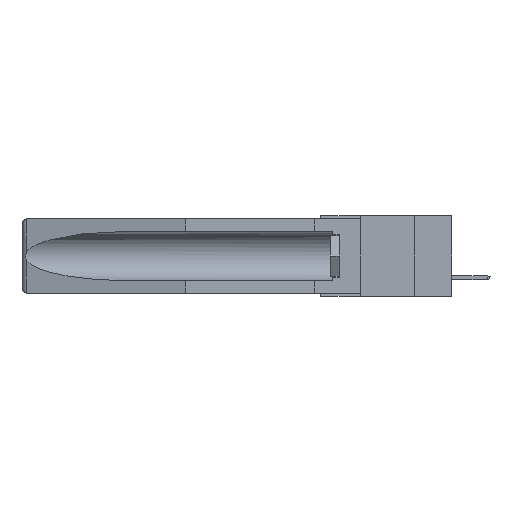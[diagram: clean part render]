
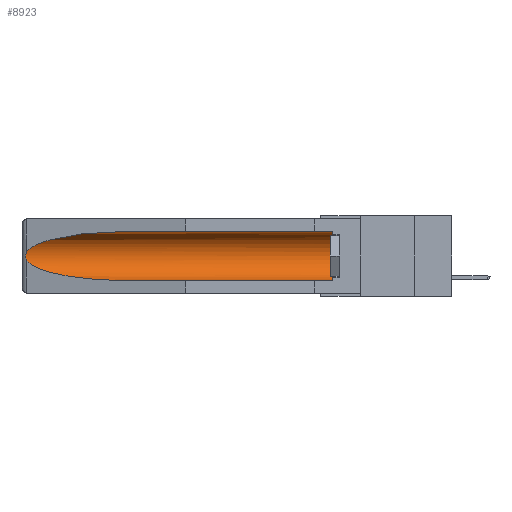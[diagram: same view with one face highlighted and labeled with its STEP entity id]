
A CAD part, left-side view. The second image highlights one B-rep face of the part: STEP entity #8923.
In plain terms, the highlighted cylindrical face has radius 2.857 mm (diameter 5.715 mm), a partial arc.
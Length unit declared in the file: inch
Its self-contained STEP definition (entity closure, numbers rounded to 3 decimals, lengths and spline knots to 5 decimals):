
#1051 = CARTESIAN_POINT ( 'NONE',  ( 0.2673, 1.5327, -0.16383 ) ) ;
#2566 = LINE ( 'NONE', #21143, #23350 ) ;
#3014 = VERTEX_POINT ( 'NONE', #20206 ) ;
#3257 = CARTESIAN_POINT ( 'NONE',  ( 0.26537, 1.52718, -0.19328 ) ) ;
#3435 = CARTESIAN_POINT ( 'NONE',  ( 0.26537, 1.52718, -0.14972 ) ) ;
#4205 = CARTESIAN_POINT ( 'NONE',  ( 0.26537, 1.52718, -0.14972 ) ) ;
#4552 = ORIENTED_EDGE ( 'NONE', *, *, #18517, .T. ) ;
#4690 = VERTEX_POINT ( 'NONE', #9397 ) ;
#5372 = CARTESIAN_POINT ( 'NONE',  ( 0.155, 0.126, -0.059 ) ) ;
#5679 = CARTESIAN_POINT ( 'NONE',  ( 0.26597, 1.5296, -0.19026 ) ) ;
#5900 = DIRECTION ( 'NONE',  ( 0., 1., 0. ) ) ;
#6109 = AXIS2_PLACEMENT_3D ( 'NONE', #16629, #5900, #23054 ) ;
#6149 = AXIS2_PLACEMENT_3D ( 'NONE', #6812, #26758, #14187 ) ;
#6570 = CARTESIAN_POINT ( 'NONE',  ( 0.155, 1.07973, -0.284 ) ) ;
#6812 = CARTESIAN_POINT ( 'NONE',  ( 0.155, 0.126, -0.1715 ) ) ;
#7363 = CARTESIAN_POINT ( 'NONE',  ( 0.26597, 1.52961, -0.15275 ) ) ;
#7870 = VERTEX_POINT ( 'NONE', #6570 ) ;
#7963 = VERTEX_POINT ( 'NONE', #15743 ) ;
#8196 =( BOUNDED_CURVE ( )  B_SPLINE_CURVE ( 3, ( #14705, #23470, #21165, #4205 ),
 .UNSPECIFIED., .F., .F. ) 
 B_SPLINE_CURVE_WITH_KNOTS ( ( 4, 4 ),
 ( 4.71239, 6.08839 ),
 .UNSPECIFIED. ) 
 CURVE ( )  GEOMETRIC_REPRESENTATION_ITEM ( )  RATIONAL_B_SPLINE_CURVE ( ( 1., 0.848, 0.848, 1. ) ) 
 REPRESENTATION_ITEM ( '' )  );
#8923 = ADVANCED_FACE ( 'NONE', ( #19555 ), #13847, .F. ) ;
#9397 = CARTESIAN_POINT ( 'NONE',  ( 0.155, 0.126, -0.284 ) ) ;
#9879 = CARTESIAN_POINT ( 'NONE',  ( 0.2675, 1.53308, -0.16763 ) ) ;
#10232 = EDGE_LOOP ( 'NONE', ( #20645, #14268, #4552, #20468, #12966, #24654 ) ) ;
#11658 = EDGE_CURVE ( 'NONE', #4690, #19636, #20367, .T. ) ;
#12394 = CARTESIAN_POINT ( 'NONE',  ( 0.25451, 1.48313, -0.24835 ) ) ;
#12966 = ORIENTED_EDGE ( 'NONE', *, *, #11658, .T. ) ;
#13592 = VECTOR ( 'NONE', #20528, 39.37008 ) ;
#13847 = CYLINDRICAL_SURFACE ( 'NONE', #6109, 0.1125 ) ;
#14187 = DIRECTION ( 'NONE',  ( 0., 0., 1. ) ) ;
#14268 = ORIENTED_EDGE ( 'NONE', *, *, #18723, .T. ) ;
#14344 = CARTESIAN_POINT ( 'NONE',  ( 0.155, -0.30754, -0.059 ) ) ;
#14534 = CARTESIAN_POINT ( 'NONE',  ( 0.155, 1.07973, -0.284 ) ) ;
#14582 = EDGE_CURVE ( 'NONE', #3014, #7963, #8196, .T. ) ;
#14705 = CARTESIAN_POINT ( 'NONE',  ( 0.155, 1.07973, -0.059 ) ) ;
#15743 = CARTESIAN_POINT ( 'NONE',  ( 0.26537, 1.52718, -0.14972 ) ) ;
#15986 = EDGE_CURVE ( 'NONE', #19636, #3014, #27618, .T. ) ;
#16610 = VERTEX_POINT ( 'NONE', #25281 ) ;
#16629 = CARTESIAN_POINT ( 'NONE',  ( 0.155, -0.30754, -0.1715 ) ) ;
#16876 = DIRECTION ( 'NONE',  ( 0., 1., 0. ) ) ;
#18517 = EDGE_CURVE ( 'NONE', #16610, #7870, #27719, .T. ) ;
#18723 = EDGE_CURVE ( 'NONE', #7963, #16610, #22783, .T. ) ;
#19555 = FACE_OUTER_BOUND ( 'NONE', #10232, .T. ) ;
#19636 = VERTEX_POINT ( 'NONE', #5372 ) ;
#20206 = CARTESIAN_POINT ( 'NONE',  ( 0.155, 1.07973, -0.059 ) ) ;
#20367 = CIRCLE ( 'NONE', #6149, 0.1125 ) ;
#20468 = ORIENTED_EDGE ( 'NONE', *, *, #21219, .F. ) ;
#20528 = DIRECTION ( 'NONE',  ( 0., 1., 0. ) ) ;
#20645 = ORIENTED_EDGE ( 'NONE', *, *, #14582, .T. ) ;
#20711 = CARTESIAN_POINT ( 'NONE',  ( 0.26537, 1.52718, -0.19328 ) ) ;
#20799 = CARTESIAN_POINT ( 'NONE',  ( 0.21114, 1.30732, -0.284 ) ) ;
#21143 = CARTESIAN_POINT ( 'NONE',  ( 0.155, -0.30754, -0.284 ) ) ;
#21165 = CARTESIAN_POINT ( 'NONE',  ( 0.25451, 1.48313, -0.09465 ) ) ;
#21219 = EDGE_CURVE ( 'NONE', #4690, #7870, #2566, .T. ) ;
#22440 = CARTESIAN_POINT ( 'NONE',  ( 0.26655, 1.53094, -0.18657 ) ) ;
#22535 = CARTESIAN_POINT ( 'NONE',  ( 0.2675, 1.53308, -0.17534 ) ) ;
#22713 = CARTESIAN_POINT ( 'NONE',  ( 0.26654, 1.53092, -0.15636 ) ) ;
#22783 = B_SPLINE_CURVE_WITH_KNOTS ( 'NONE', 3,
 ( #3435, #7363, #22713, #1051, #9879, #22535, #26976, #22440, #5679, #3257 ),
 .UNSPECIFIED., .F., .F.,
 ( 4, 2, 2, 2, 4 ),
 ( 0., 0.00029, 0.00058, 0.00087, 0.00117 ),
 .UNSPECIFIED. ) ;
#23054 = DIRECTION ( 'NONE',  ( 0., 0., 1. ) ) ;
#23350 = VECTOR ( 'NONE', #16876, 39.37008 ) ;
#23470 = CARTESIAN_POINT ( 'NONE',  ( 0.21114, 1.30732, -0.059 ) ) ;
#24654 = ORIENTED_EDGE ( 'NONE', *, *, #15986, .T. ) ;
#25281 = CARTESIAN_POINT ( 'NONE',  ( 0.26537, 1.52718, -0.19328 ) ) ;
#26758 = DIRECTION ( 'NONE',  ( 0., -1., 0. ) ) ;
#26976 = CARTESIAN_POINT ( 'NONE',  ( 0.2673, 1.53269, -0.17917 ) ) ;
#27618 = LINE ( 'NONE', #14344, #13592 ) ;
#27719 =( BOUNDED_CURVE ( )  B_SPLINE_CURVE ( 3, ( #20711, #12394, #20799, #14534 ),
 .UNSPECIFIED., .F., .F. ) 
 B_SPLINE_CURVE_WITH_KNOTS ( ( 4, 4 ),
 ( 0.1948, 1.5708 ),
 .UNSPECIFIED. ) 
 CURVE ( )  GEOMETRIC_REPRESENTATION_ITEM ( )  RATIONAL_B_SPLINE_CURVE ( ( 1., 0.848, 0.848, 1. ) ) 
 REPRESENTATION_ITEM ( '' )  );
